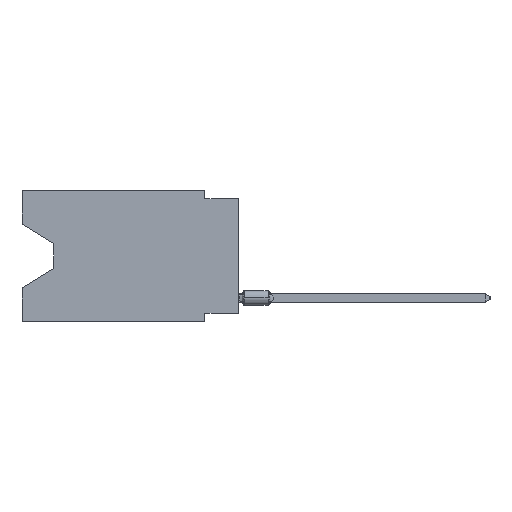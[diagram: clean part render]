
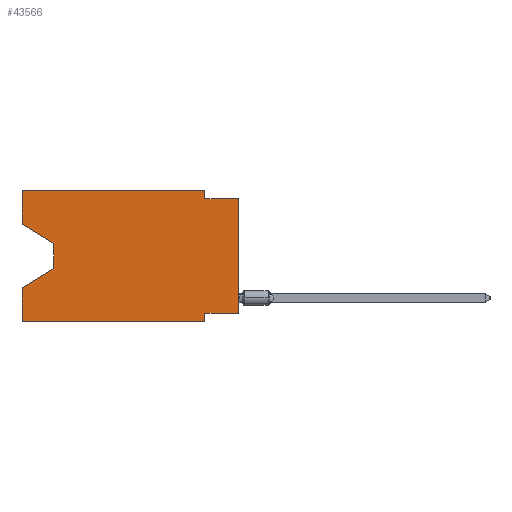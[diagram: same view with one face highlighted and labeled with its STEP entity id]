
A CAD part, left-side view. The second image highlights one B-rep face of the part: STEP entity #43566.
In plain terms, the highlighted planar face has unit normal (-1, 0, 0).
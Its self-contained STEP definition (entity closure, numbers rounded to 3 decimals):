
#822 = VECTOR ( 'NONE', #45176, 1000. ) ;
#1658 = VERTEX_POINT ( 'NONE', #47562 ) ;
#1847 = EDGE_CURVE ( 'NONE', #8431, #13487, #30129, .T. ) ;
#2076 = VECTOR ( 'NONE', #29657, 1000. ) ;
#5044 = CARTESIAN_POINT ( 'NONE',  ( 0., 0., -0.635 ) ) ;
#5566 = DIRECTION ( 'NONE',  ( 0., 0., -1. ) ) ;
#5601 = VECTOR ( 'NONE', #19361, 1000. ) ;
#8431 = VERTEX_POINT ( 'NONE', #47088 ) ;
#8999 = DIRECTION ( 'NONE',  ( 1., 0., 0. ) ) ;
#9101 = VERTEX_POINT ( 'NONE', #55654 ) ;
#10270 = LINE ( 'NONE', #19136, #27229 ) ;
#10918 = CARTESIAN_POINT ( 'NONE',  ( 0., 16.383, -2.546 ) ) ;
#11496 = EDGE_CURVE ( 'NONE', #23639, #46414, #61609, .T. ) ;
#13266 = EDGE_LOOP ( 'NONE', ( #35511, #43695, #25748, #25856, #23169, #31776, #50427, #50851, #16773, #26618, #32136, #34767 ) ) ;
#13487 = VERTEX_POINT ( 'NONE', #37554 ) ;
#14448 = DIRECTION ( 'NONE',  ( 0., -1., 0. ) ) ;
#15646 = CARTESIAN_POINT ( 'NONE',  ( 0., 0., -0.635 ) ) ;
#16773 = ORIENTED_EDGE ( 'NONE', *, *, #64177, .F. ) ;
#17526 = VECTOR ( 'NONE', #5566, 1000. ) ;
#17978 = VERTEX_POINT ( 'NONE', #5044 ) ;
#18482 = CARTESIAN_POINT ( 'NONE',  ( 0., 0., -9.271 ) ) ;
#18817 = CARTESIAN_POINT ( 'NONE',  ( 0., 16.383, 0. ) ) ;
#19136 = CARTESIAN_POINT ( 'NONE',  ( 0., 0., 0. ) ) ;
#19361 = DIRECTION ( 'NONE',  ( 0., 0., -1. ) ) ;
#21588 = LINE ( 'NONE', #37002, #51803 ) ;
#21699 = CARTESIAN_POINT ( 'NONE',  ( 0., 0., -9.271 ) ) ;
#21919 = CARTESIAN_POINT ( 'NONE',  ( 0., 13.97, -4.013 ) ) ;
#22598 = EDGE_CURVE ( 'NONE', #22699, #9101, #33480, .T. ) ;
#22699 = VERTEX_POINT ( 'NONE', #36379 ) ;
#23169 = ORIENTED_EDGE ( 'NONE', *, *, #40983, .T. ) ;
#23639 = VERTEX_POINT ( 'NONE', #10918 ) ;
#24282 = CARTESIAN_POINT ( 'NONE',  ( 0., 2.54, 0. ) ) ;
#24867 = DIRECTION ( 'NONE',  ( 0., 0.855, -0.519 ) ) ;
#25020 = VERTEX_POINT ( 'NONE', #18482 ) ;
#25155 = LINE ( 'NONE', #15646, #822 ) ;
#25748 = ORIENTED_EDGE ( 'NONE', *, *, #1847, .T. ) ;
#25856 = ORIENTED_EDGE ( 'NONE', *, *, #32040, .F. ) ;
#26540 = VECTOR ( 'NONE', #24867, 1000. ) ;
#26618 = ORIENTED_EDGE ( 'NONE', *, *, #22598, .F. ) ;
#27198 = CARTESIAN_POINT ( 'NONE',  ( 0., 13.97, -4.013 ) ) ;
#27229 = VECTOR ( 'NONE', #55198, 1000. ) ;
#28568 = CARTESIAN_POINT ( 'NONE',  ( 0., 16.383, 0. ) ) ;
#29002 = DIRECTION ( 'NONE',  ( 0., 0., -1. ) ) ;
#29217 = LINE ( 'NONE', #28568, #30885 ) ;
#29657 = DIRECTION ( 'NONE',  ( 0., -1., 0. ) ) ;
#29687 = CARTESIAN_POINT ( 'NONE',  ( 0., 2.54, -9.271 ) ) ;
#30129 = LINE ( 'NONE', #50137, #26540 ) ;
#30613 = VERTEX_POINT ( 'NONE', #43810 ) ;
#30885 = VECTOR ( 'NONE', #14448, 1000. ) ;
#31158 = EDGE_CURVE ( 'NONE', #25020, #17978, #10270, .T. ) ;
#31464 = LINE ( 'NONE', #62295, #61832 ) ;
#31776 = ORIENTED_EDGE ( 'NONE', *, *, #35958, .F. ) ;
#32040 = EDGE_CURVE ( 'NONE', #30613, #13487, #31464, .T. ) ;
#32070 = CARTESIAN_POINT ( 'NONE',  ( 0., 16.383, 0. ) ) ;
#32136 = ORIENTED_EDGE ( 'NONE', *, *, #61740, .F. ) ;
#33480 = LINE ( 'NONE', #24282, #59430 ) ;
#33907 = FACE_OUTER_BOUND ( 'NONE', #13266, .T. ) ;
#34431 = CARTESIAN_POINT ( 'NONE',  ( 0., 2.54, -9.906 ) ) ;
#34767 = ORIENTED_EDGE ( 'NONE', *, *, #11496, .F. ) ;
#35508 = LINE ( 'NONE', #21699, #43167 ) ;
#35511 = ORIENTED_EDGE ( 'NONE', *, *, #37865, .T. ) ;
#35958 = EDGE_CURVE ( 'NONE', #43648, #1658, #64612, .T. ) ;
#36031 = DIRECTION ( 'NONE',  ( 0., 0., 1. ) ) ;
#36379 = CARTESIAN_POINT ( 'NONE',  ( 0., 2.54, 0. ) ) ;
#37002 = CARTESIAN_POINT ( 'NONE',  ( 0., 16.383, -2.546 ) ) ;
#37554 = CARTESIAN_POINT ( 'NONE',  ( 0., 16.383, -7.36 ) ) ;
#37865 = EDGE_CURVE ( 'NONE', #23639, #46252, #21588, .T. ) ;
#39905 = VECTOR ( 'NONE', #36031, 1000. ) ;
#40983 = EDGE_CURVE ( 'NONE', #30613, #1658, #63471, .T. ) ;
#43167 = VECTOR ( 'NONE', #60774, 1000. ) ;
#43566 = ADVANCED_FACE ( 'NONE', ( #33907 ), #53919, .F. ) ;
#43648 = VERTEX_POINT ( 'NONE', #29687 ) ;
#43695 = ORIENTED_EDGE ( 'NONE', *, *, #63818, .T. ) ;
#43810 = CARTESIAN_POINT ( 'NONE',  ( 0., 16.383, -9.906 ) ) ;
#45176 = DIRECTION ( 'NONE',  ( 0., -1., 0. ) ) ;
#45401 = EDGE_CURVE ( 'NONE', #25020, #43648, #35508, .T. ) ;
#46252 = VERTEX_POINT ( 'NONE', #27198 ) ;
#46414 = VERTEX_POINT ( 'NONE', #51638 ) ;
#47088 = CARTESIAN_POINT ( 'NONE',  ( 0., 13.97, -5.893 ) ) ;
#47562 = CARTESIAN_POINT ( 'NONE',  ( 0., 2.54, -9.906 ) ) ;
#49878 = DIRECTION ( 'NONE',  ( 0., 0., -1. ) ) ;
#50137 = CARTESIAN_POINT ( 'NONE',  ( 0., 13.97, -5.893 ) ) ;
#50427 = ORIENTED_EDGE ( 'NONE', *, *, #45401, .F. ) ;
#50851 = ORIENTED_EDGE ( 'NONE', *, *, #31158, .T. ) ;
#51140 = LINE ( 'NONE', #21919, #17526 ) ;
#51456 = DIRECTION ( 'NONE',  ( 0., -0.855, -0.519 ) ) ;
#51638 = CARTESIAN_POINT ( 'NONE',  ( 0., 16.383, 0. ) ) ;
#51792 = DIRECTION ( 'NONE',  ( 0., 0., 1. ) ) ;
#51803 = VECTOR ( 'NONE', #51456, 1000. ) ;
#53919 = PLANE ( 'NONE',  #62051 ) ;
#53946 = CARTESIAN_POINT ( 'NONE',  ( 0., 16.383, -9.906 ) ) ;
#55198 = DIRECTION ( 'NONE',  ( 0., 0., 1. ) ) ;
#55654 = CARTESIAN_POINT ( 'NONE',  ( 0., 2.54, -0.635 ) ) ;
#59430 = VECTOR ( 'NONE', #49878, 1000. ) ;
#60774 = DIRECTION ( 'NONE',  ( 0., 1., 0. ) ) ;
#61609 = LINE ( 'NONE', #32070, #39905 ) ;
#61740 = EDGE_CURVE ( 'NONE', #46414, #22699, #29217, .T. ) ;
#61832 = VECTOR ( 'NONE', #51792, 1000. ) ;
#62051 = AXIS2_PLACEMENT_3D ( 'NONE', #18817, #8999, #29002 ) ;
#62295 = CARTESIAN_POINT ( 'NONE',  ( 0., 16.383, 0. ) ) ;
#63471 = LINE ( 'NONE', #53946, #2076 ) ;
#63818 = EDGE_CURVE ( 'NONE', #46252, #8431, #51140, .T. ) ;
#64177 = EDGE_CURVE ( 'NONE', #9101, #17978, #25155, .T. ) ;
#64612 = LINE ( 'NONE', #34431, #5601 ) ;
